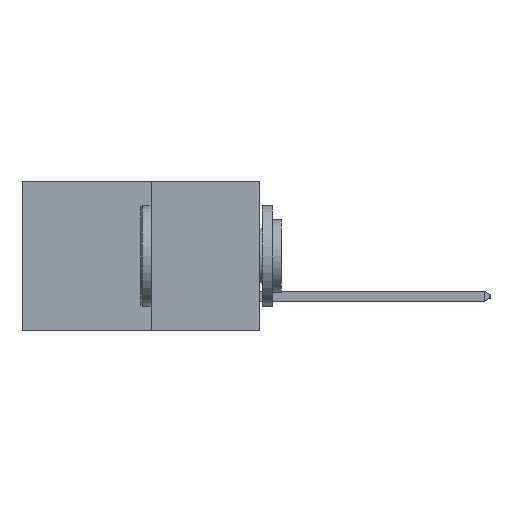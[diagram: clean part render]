
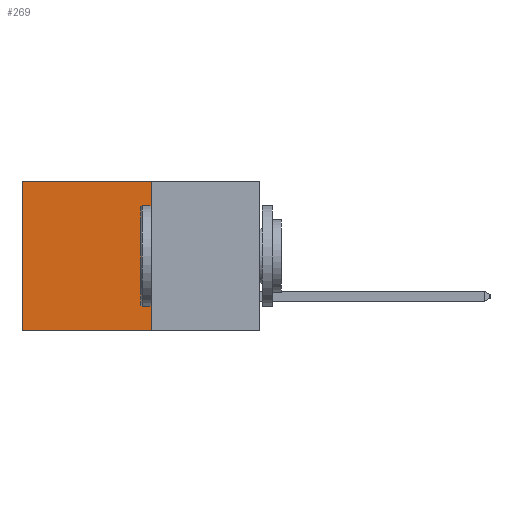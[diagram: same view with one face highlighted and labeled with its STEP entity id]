
A CAD part, left-side view. The second image highlights one B-rep face of the part: STEP entity #269.
In plain terms, the highlighted planar face has unit normal (-1, 0, 0).
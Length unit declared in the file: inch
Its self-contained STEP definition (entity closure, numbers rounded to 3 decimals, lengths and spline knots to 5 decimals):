
#218 = VERTEX_POINT ( 'NONE', #18238 ) ;
#268 = EDGE_CURVE ( 'NONE', #11016, #11374, #12860, .T. ) ;
#269 = ADVANCED_FACE ( 'NONE', ( #16915 ), #5730, .F. ) ;
#637 = EDGE_CURVE ( 'NONE', #11374, #218, #9884, .T. ) ;
#868 = CARTESIAN_POINT ( 'NONE',  ( 0.277, 0.59, 0. ) ) ;
#2264 = CARTESIAN_POINT ( 'NONE',  ( 0.277, 0.59, -0.37 ) ) ;
#2265 = ORIENTED_EDGE ( 'NONE', *, *, #6792, .F. ) ;
#2967 = ORIENTED_EDGE ( 'NONE', *, *, #268, .T. ) ;
#2993 = AXIS2_PLACEMENT_3D ( 'NONE', #6118, #12011, #11954 ) ;
#5177 = VECTOR ( 'NONE', #17884, 39.37008 ) ;
#5730 = PLANE ( 'NONE',  #2993 ) ;
#5805 = EDGE_LOOP ( 'NONE', ( #9022, #9480, #2265, #2967 ) ) ;
#6013 = CARTESIAN_POINT ( 'NONE',  ( 0.277, 0.27, 0. ) ) ;
#6091 = CARTESIAN_POINT ( 'NONE',  ( 0.277, 0.27, -0.37 ) ) ;
#6109 = DIRECTION ( 'NONE',  ( 0., 1., 0. ) ) ;
#6118 = CARTESIAN_POINT ( 'NONE',  ( 0.277, 0.27, -0.37 ) ) ;
#6247 = LINE ( 'NONE', #13815, #13870 ) ;
#6774 = DIRECTION ( 'NONE',  ( 0., 0., -1. ) ) ;
#6792 = EDGE_CURVE ( 'NONE', #11016, #13673, #6247, .T. ) ;
#7385 = VECTOR ( 'NONE', #6109, 39.37008 ) ;
#7715 = CARTESIAN_POINT ( 'NONE',  ( 0.277, 0.27, -0.37 ) ) ;
#9022 = ORIENTED_EDGE ( 'NONE', *, *, #637, .T. ) ;
#9274 = EDGE_CURVE ( 'NONE', #13673, #218, #11701, .T. ) ;
#9480 = ORIENTED_EDGE ( 'NONE', *, *, #9274, .F. ) ;
#9884 = LINE ( 'NONE', #2264, #13271 ) ;
#11016 = VERTEX_POINT ( 'NONE', #15798 ) ;
#11374 = VERTEX_POINT ( 'NONE', #868 ) ;
#11701 = LINE ( 'NONE', #6091, #7385 ) ;
#11954 = DIRECTION ( 'NONE',  ( 0., 0., -1. ) ) ;
#12011 = DIRECTION ( 'NONE',  ( 1., 0., 0. ) ) ;
#12860 = LINE ( 'NONE', #6013, #5177 ) ;
#13271 = VECTOR ( 'NONE', #6774, 39.37008 ) ;
#13464 = DIRECTION ( 'NONE',  ( 0., 0., -1. ) ) ;
#13673 = VERTEX_POINT ( 'NONE', #7715 ) ;
#13815 = CARTESIAN_POINT ( 'NONE',  ( 0.277, 0.27, -0.37 ) ) ;
#13870 = VECTOR ( 'NONE', #13464, 39.37008 ) ;
#15798 = CARTESIAN_POINT ( 'NONE',  ( 0.277, 0.27, 0. ) ) ;
#16915 = FACE_OUTER_BOUND ( 'NONE', #5805, .T. ) ;
#17884 = DIRECTION ( 'NONE',  ( 0., 1., 0. ) ) ;
#18238 = CARTESIAN_POINT ( 'NONE',  ( 0.277, 0.59, -0.37 ) ) ;
